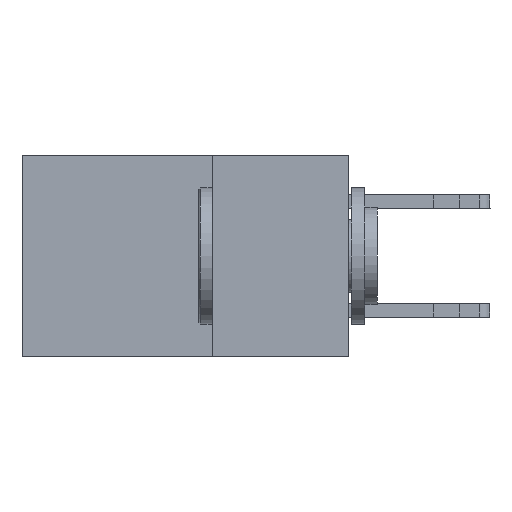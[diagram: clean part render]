
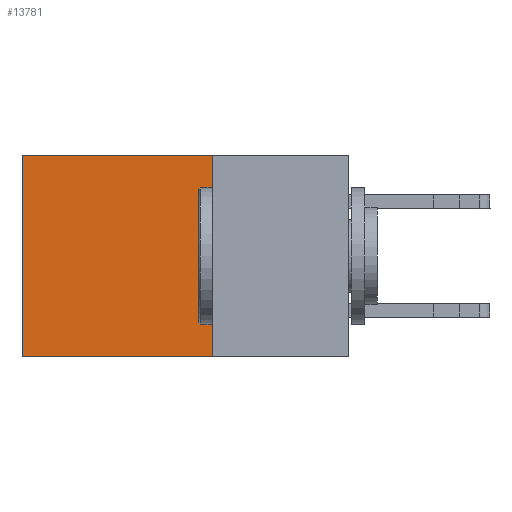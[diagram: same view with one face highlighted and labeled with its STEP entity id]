
A CAD part, left-side view. The second image highlights one B-rep face of the part: STEP entity #13781.
In plain terms, the highlighted planar face has unit normal (-1, 0, 0).
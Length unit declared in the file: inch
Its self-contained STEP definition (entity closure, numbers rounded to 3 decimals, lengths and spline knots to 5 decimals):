
#258 = CARTESIAN_POINT ( 'NONE',  ( 0.298, 0.25, 0. ) ) ;
#606 = CARTESIAN_POINT ( 'NONE',  ( 0.298, 0.25, 0. ) ) ;
#663 = VERTEX_POINT ( 'NONE', #10802 ) ;
#1853 = CARTESIAN_POINT ( 'NONE',  ( 0.298, 0.25, -0.37 ) ) ;
#2068 = CARTESIAN_POINT ( 'NONE',  ( 0.298, 0.25, -0.37 ) ) ;
#2097 = EDGE_CURVE ( 'NONE', #4051, #663, #9629, .T. ) ;
#2686 = DIRECTION ( 'NONE',  ( 0., 0., -1. ) ) ;
#3290 = CARTESIAN_POINT ( 'NONE',  ( 0.298, 0.25, 0. ) ) ;
#3770 = FACE_OUTER_BOUND ( 'NONE', #13957, .T. ) ;
#3962 = EDGE_CURVE ( 'NONE', #9189, #4051, #5203, .T. ) ;
#4051 = VERTEX_POINT ( 'NONE', #2068 ) ;
#4500 = EDGE_CURVE ( 'NONE', #9189, #9000, #12044, .T. ) ;
#4690 = ORIENTED_EDGE ( 'NONE', *, *, #12674, .T. ) ;
#4719 = DIRECTION ( 'NONE',  ( 1., 0., 0. ) ) ;
#5099 = ORIENTED_EDGE ( 'NONE', *, *, #4500, .T. ) ;
#5203 = LINE ( 'NONE', #606, #10530 ) ;
#6617 = VECTOR ( 'NONE', #13395, 39.37008 ) ;
#7725 = ORIENTED_EDGE ( 'NONE', *, *, #2097, .F. ) ;
#8881 = LINE ( 'NONE', #9930, #6617 ) ;
#9000 = VERTEX_POINT ( 'NONE', #9788 ) ;
#9189 = VERTEX_POINT ( 'NONE', #10075 ) ;
#9629 = LINE ( 'NONE', #1853, #13569 ) ;
#9788 = CARTESIAN_POINT ( 'NONE',  ( 0.298, 0.6, 0. ) ) ;
#9930 = CARTESIAN_POINT ( 'NONE',  ( 0.298, 0.6, 0. ) ) ;
#10075 = CARTESIAN_POINT ( 'NONE',  ( 0.298, 0.25, 0. ) ) ;
#10530 = VECTOR ( 'NONE', #10759, 39.37008 ) ;
#10759 = DIRECTION ( 'NONE',  ( 0., 0., -1. ) ) ;
#10802 = CARTESIAN_POINT ( 'NONE',  ( 0.298, 0.6, -0.37 ) ) ;
#12044 = LINE ( 'NONE', #3290, #12444 ) ;
#12136 = ORIENTED_EDGE ( 'NONE', *, *, #3962, .F. ) ;
#12264 = DIRECTION ( 'NONE',  ( 0., 1., 0. ) ) ;
#12444 = VECTOR ( 'NONE', #12264, 39.37008 ) ;
#12674 = EDGE_CURVE ( 'NONE', #9000, #663, #8881, .T. ) ;
#12675 = PLANE ( 'NONE',  #13380 ) ;
#13380 = AXIS2_PLACEMENT_3D ( 'NONE', #258, #4719, #2686 ) ;
#13395 = DIRECTION ( 'NONE',  ( 0., 0., -1. ) ) ;
#13569 = VECTOR ( 'NONE', #14123, 39.37008 ) ;
#13781 = ADVANCED_FACE ( 'NONE', ( #3770 ), #12675, .F. ) ;
#13957 = EDGE_LOOP ( 'NONE', ( #4690, #7725, #12136, #5099 ) ) ;
#14123 = DIRECTION ( 'NONE',  ( 0., 1., 0. ) ) ;
